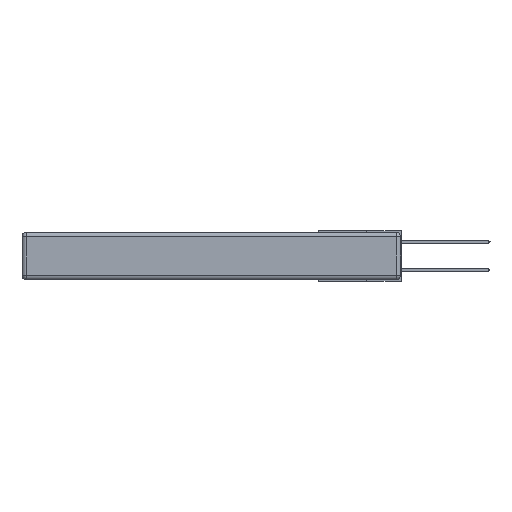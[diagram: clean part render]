
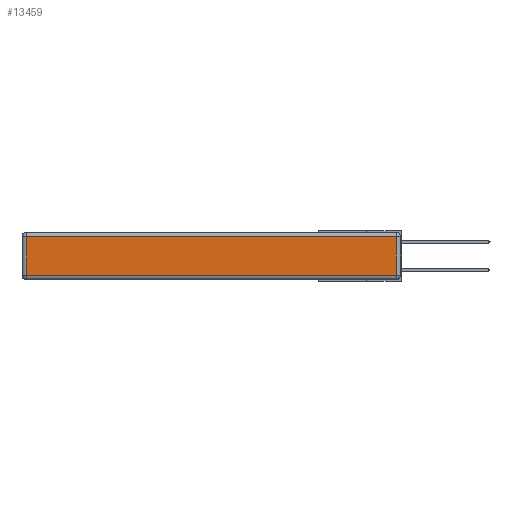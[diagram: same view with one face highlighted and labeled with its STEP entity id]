
A CAD part, left-side view. The second image highlights one B-rep face of the part: STEP entity #13459.
In plain terms, the highlighted planar face has unit normal (-1, 0, 0).
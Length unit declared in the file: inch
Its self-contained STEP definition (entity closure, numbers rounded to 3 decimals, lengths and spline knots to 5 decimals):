
#137 = CARTESIAN_POINT ( 'NONE',  ( 0., 0.03, -0.343 ) ) ;
#279 = ORIENTED_EDGE ( 'NONE', *, *, #3938, .T. ) ;
#519 = FACE_OUTER_BOUND ( 'NONE', #2480, .T. ) ;
#569 = CARTESIAN_POINT ( 'NONE',  ( 0., 0., -0.313 ) ) ;
#1485 = DIRECTION ( 'NONE',  ( 0., 0., 1. ) ) ;
#2268 = DIRECTION ( 'NONE',  ( 0., 1., 0. ) ) ;
#2480 = EDGE_LOOP ( 'NONE', ( #7852, #10056, #279, #5029 ) ) ;
#3938 = EDGE_CURVE ( 'NONE', #4756, #8653, #8094, .T. ) ;
#4756 = VERTEX_POINT ( 'NONE', #13147 ) ;
#4810 = LINE ( 'NONE', #569, #10238 ) ;
#5029 = ORIENTED_EDGE ( 'NONE', *, *, #12742, .T. ) ;
#6625 = VECTOR ( 'NONE', #12444, 39.37008 ) ;
#6958 = DIRECTION ( 'NONE',  ( 0., 0., 1. ) ) ;
#7256 = CARTESIAN_POINT ( 'NONE',  ( 0., 0.03, -0.313 ) ) ;
#7424 = VERTEX_POINT ( 'NONE', #7256 ) ;
#7435 = EDGE_CURVE ( 'NONE', #8928, #7424, #4810, .T. ) ;
#7852 = ORIENTED_EDGE ( 'NONE', *, *, #7435, .T. ) ;
#7868 = VECTOR ( 'NONE', #2268, 39.37008 ) ;
#8094 = LINE ( 'NONE', #12947, #7868 ) ;
#8653 = VERTEX_POINT ( 'NONE', #11400 ) ;
#8928 = VERTEX_POINT ( 'NONE', #11902 ) ;
#9665 = CARTESIAN_POINT ( 'NONE',  ( 0., 2.72, -0.343 ) ) ;
#10056 = ORIENTED_EDGE ( 'NONE', *, *, #15513, .T. ) ;
#10199 = LINE ( 'NONE', #9665, #6625 ) ;
#10238 = VECTOR ( 'NONE', #13944, 39.37008 ) ;
#11400 = CARTESIAN_POINT ( 'NONE',  ( 0., 2.72, -0.03 ) ) ;
#11840 = VECTOR ( 'NONE', #1485, 39.37008 ) ;
#11902 = CARTESIAN_POINT ( 'NONE',  ( 0., 2.72, -0.313 ) ) ;
#12444 = DIRECTION ( 'NONE',  ( 0., 0., -1. ) ) ;
#12742 = EDGE_CURVE ( 'NONE', #8653, #8928, #10199, .T. ) ;
#12947 = CARTESIAN_POINT ( 'NONE',  ( 0., 2.75, -0.03 ) ) ;
#13147 = CARTESIAN_POINT ( 'NONE',  ( 0., 0.03, -0.03 ) ) ;
#13459 = ADVANCED_FACE ( 'NONE', ( #519 ), #14888, .T. ) ;
#13604 = CARTESIAN_POINT ( 'NONE',  ( 0., 0., -0.343 ) ) ;
#13944 = DIRECTION ( 'NONE',  ( 0., -1., 0. ) ) ;
#14888 = PLANE ( 'NONE',  #17157 ) ;
#14948 = DIRECTION ( 'NONE',  ( -1., 0., 0. ) ) ;
#15513 = EDGE_CURVE ( 'NONE', #7424, #4756, #16215, .T. ) ;
#16215 = LINE ( 'NONE', #137, #11840 ) ;
#17157 = AXIS2_PLACEMENT_3D ( 'NONE', #13604, #14948, #6958 ) ;
